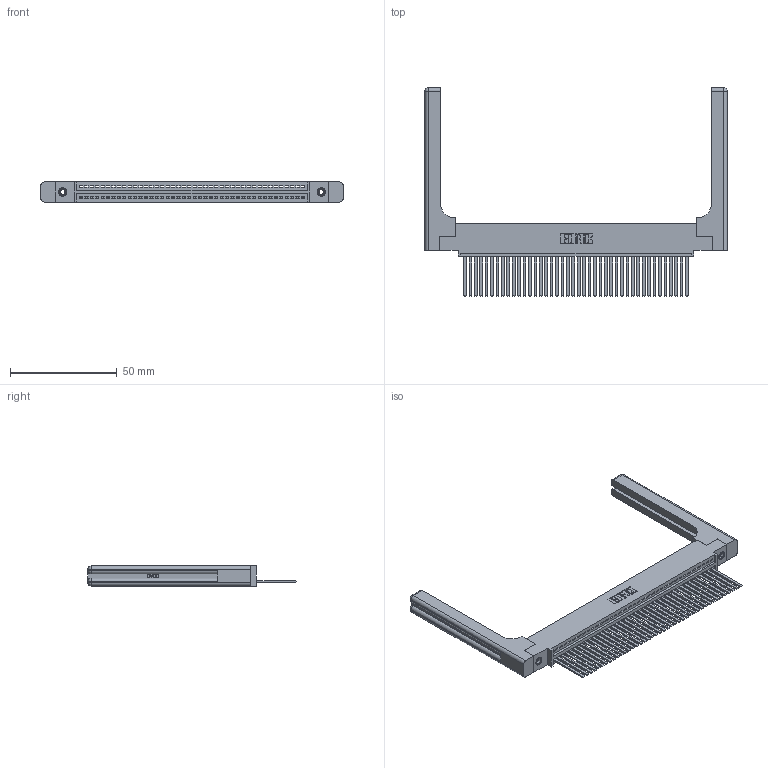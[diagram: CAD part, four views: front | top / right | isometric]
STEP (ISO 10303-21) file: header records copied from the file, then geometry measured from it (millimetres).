
FILE_DESCRIPTION (( 'STEP AP203' ), '1' );
FILE_NAME ('395-042-544-458.STEP', '2019-10-22T12:58:32', ( '' ), ( '' ), 'SwSTEP 2.0', 'SolidWorks 2016', '' );
FILE_SCHEMA (( 'CONFIG_CONTROL_DESIGN' ));
Length unit declared in the file: inch
Products named in the file (5): 345-292-001_345-293-144; 345-220-058_345-220-058; 395-042-544-458; 345 Part_0.110 Offset - 0.156 Dia-TH; 345-250-001_345-250-001-102
Assembly tree (47 placements, depth 2):
  395-042-544-458
    345 Part_0.110 Offset - 0.156 Dia-TH
    345-292-001_345-293-144  x42
    345-250-001_345-250-001-102  x2
    345-220-058_345-220-058  x2
Bounding box: 141.71 x 97.71 x 9.4 mm (x, y, z)
Volume: 22377.4 mm3; surface area: 25283 mm2
Topology: 47 solids, 47 shells, 2570 faces, 7655 edges, 5026 vertices
Faces by surface type: plane 1744, cylinder 766, bspline 36, cone 12, sphere 8, torus 4
Entity records: 36740 total; most frequent: CARTESIAN_POINT 7335, ORIENTED_EDGE 6108, DIRECTION 5350, EDGE_CURVE 3054, LINE 2666, VECTOR 2666, VERTEX_POINT 2026, AXIS2_PLACEMENT_3D 1342
